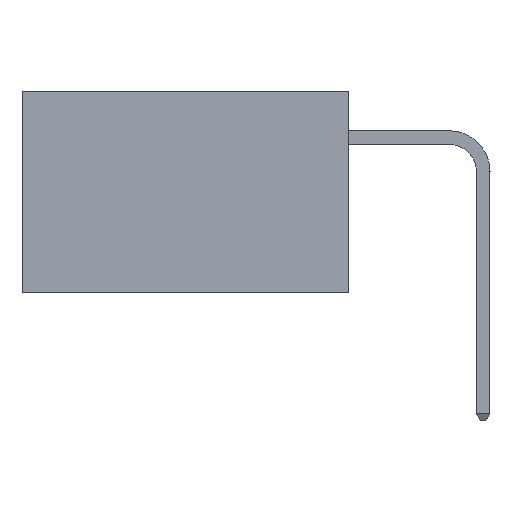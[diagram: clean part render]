
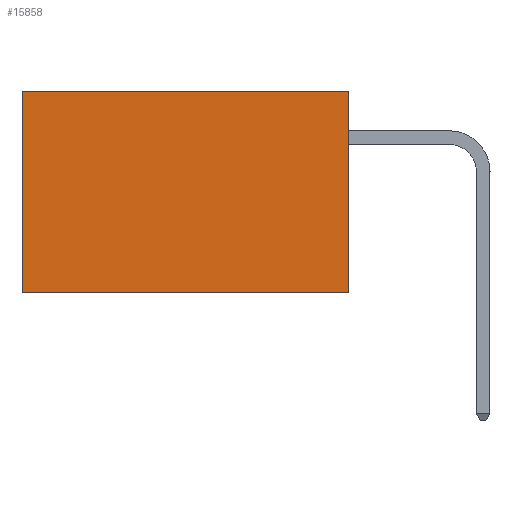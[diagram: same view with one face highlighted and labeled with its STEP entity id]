
A CAD part, left-side view. The second image highlights one B-rep face of the part: STEP entity #15858.
In plain terms, the highlighted planar face has unit normal (-1, 0, 0).
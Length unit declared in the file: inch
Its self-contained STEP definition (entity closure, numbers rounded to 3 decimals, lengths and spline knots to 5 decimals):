
#2355 = DIRECTION ( 'NONE',  ( 0., 0., -1. ) ) ;
#2699 = CARTESIAN_POINT ( 'NONE',  ( 0.2875, 0.6, -0.37 ) ) ;
#2786 = CARTESIAN_POINT ( 'NONE',  ( 0.2875, 0., 0. ) ) ;
#6266 = DIRECTION ( 'NONE',  ( 0., 1., 0. ) ) ;
#7437 = AXIS2_PLACEMENT_3D ( 'NONE', #23597, #10173, #34076 ) ;
#7829 = CARTESIAN_POINT ( 'NONE',  ( 0.2875, 0.6, 0. ) ) ;
#7985 = DIRECTION ( 'NONE',  ( 0., 0., -1. ) ) ;
#8892 = VECTOR ( 'NONE', #7985, 39.37008 ) ;
#10173 = DIRECTION ( 'NONE',  ( 1., 0., 0. ) ) ;
#10671 = ORIENTED_EDGE ( 'NONE', *, *, #43956, .T. ) ;
#13570 = VECTOR ( 'NONE', #6266, 39.37008 ) ;
#13851 = ORIENTED_EDGE ( 'NONE', *, *, #14343, .F. ) ;
#14343 = EDGE_CURVE ( 'NONE', #36122, #42576, #15801, .T. ) ;
#15297 = VECTOR ( 'NONE', #2355, 39.37008 ) ;
#15801 = LINE ( 'NONE', #25815, #32927 ) ;
#15858 = ADVANCED_FACE ( 'NONE', ( #38331 ), #30612, .F. ) ;
#16195 = CARTESIAN_POINT ( 'NONE',  ( 0.2875, 0., 0. ) ) ;
#20294 = VERTEX_POINT ( 'NONE', #27573 ) ;
#22670 = LINE ( 'NONE', #2786, #13570 ) ;
#23027 = ORIENTED_EDGE ( 'NONE', *, *, #43114, .F. ) ;
#23597 = CARTESIAN_POINT ( 'NONE',  ( 0.2875, 0., 0. ) ) ;
#25815 = CARTESIAN_POINT ( 'NONE',  ( 0.2875, 0., -0.37 ) ) ;
#25998 = LINE ( 'NONE', #7829, #8892 ) ;
#26013 = CARTESIAN_POINT ( 'NONE',  ( 0.2875, 0., -0.37 ) ) ;
#26123 = DIRECTION ( 'NONE',  ( 0., 1., 0. ) ) ;
#27573 = CARTESIAN_POINT ( 'NONE',  ( 0.2875, 0.6, 0. ) ) ;
#30612 = PLANE ( 'NONE',  #7437 ) ;
#30860 = ORIENTED_EDGE ( 'NONE', *, *, #34230, .T. ) ;
#32927 = VECTOR ( 'NONE', #26123, 39.37008 ) ;
#33038 = CARTESIAN_POINT ( 'NONE',  ( 0.2875, 0., 0. ) ) ;
#33481 = LINE ( 'NONE', #33038, #15297 ) ;
#34076 = DIRECTION ( 'NONE',  ( 0., 0., -1. ) ) ;
#34230 = EDGE_CURVE ( 'NONE', #42526, #20294, #22670, .T. ) ;
#36122 = VERTEX_POINT ( 'NONE', #26013 ) ;
#37599 = EDGE_LOOP ( 'NONE', ( #10671, #13851, #23027, #30860 ) ) ;
#38331 = FACE_OUTER_BOUND ( 'NONE', #37599, .T. ) ;
#42526 = VERTEX_POINT ( 'NONE', #16195 ) ;
#42576 = VERTEX_POINT ( 'NONE', #2699 ) ;
#43114 = EDGE_CURVE ( 'NONE', #42526, #36122, #33481, .T. ) ;
#43956 = EDGE_CURVE ( 'NONE', #20294, #42576, #25998, .T. ) ;
